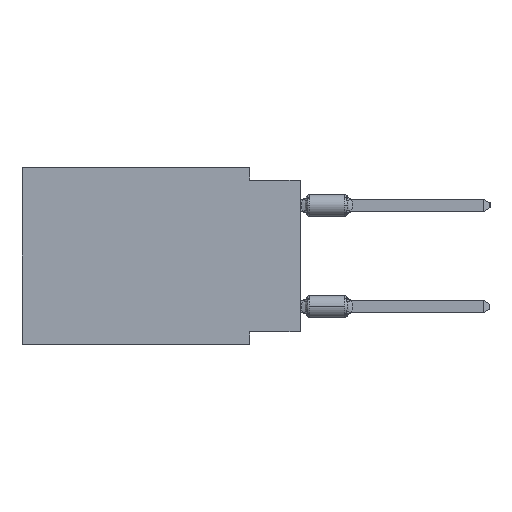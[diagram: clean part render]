
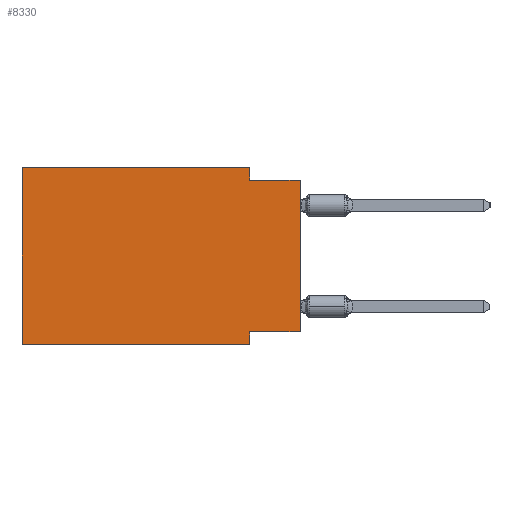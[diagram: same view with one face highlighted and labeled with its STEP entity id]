
A CAD part, left-side view. The second image highlights one B-rep face of the part: STEP entity #8330.
In plain terms, the highlighted planar face has unit normal (-1, 0, 0).
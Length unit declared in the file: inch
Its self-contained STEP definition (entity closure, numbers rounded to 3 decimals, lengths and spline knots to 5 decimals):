
#91 = LINE ( 'NONE', #12347, #8496 ) ;
#528 = VECTOR ( 'NONE', #4698, 39.37008 ) ;
#747 = ORIENTED_EDGE ( 'NONE', *, *, #12463, .F. ) ;
#889 = CARTESIAN_POINT ( 'NONE',  ( 0., 0., -0.325 ) ) ;
#1153 = VERTEX_POINT ( 'NONE', #8710 ) ;
#1393 = ORIENTED_EDGE ( 'NONE', *, *, #4732, .F. ) ;
#1495 = PLANE ( 'NONE',  #18322 ) ;
#1607 = CARTESIAN_POINT ( 'NONE',  ( 0., 0., -0.025 ) ) ;
#1635 = LINE ( 'NONE', #15175, #3743 ) ;
#1828 = CARTESIAN_POINT ( 'NONE',  ( 0., 0.1, -0.35 ) ) ;
#1936 = LINE ( 'NONE', #8005, #528 ) ;
#1984 = DIRECTION ( 'NONE',  ( 0., 0., 1. ) ) ;
#2000 = VERTEX_POINT ( 'NONE', #19093 ) ;
#2372 = CARTESIAN_POINT ( 'NONE',  ( 0., 0., -0.325 ) ) ;
#2794 = ORIENTED_EDGE ( 'NONE', *, *, #16580, .F. ) ;
#2801 = DIRECTION ( 'NONE',  ( 0., 0., -1. ) ) ;
#3112 = VERTEX_POINT ( 'NONE', #2372 ) ;
#3304 = DIRECTION ( 'NONE',  ( 0., 0., -1. ) ) ;
#3743 = VECTOR ( 'NONE', #13691, 39.37008 ) ;
#4173 = VERTEX_POINT ( 'NONE', #7600 ) ;
#4698 = DIRECTION ( 'NONE',  ( 0., 0., 1. ) ) ;
#4732 = EDGE_CURVE ( 'NONE', #1153, #16772, #4841, .T. ) ;
#4841 = LINE ( 'NONE', #10838, #7838 ) ;
#5769 = EDGE_CURVE ( 'NONE', #9960, #4173, #19409, .T. ) ;
#6175 = ORIENTED_EDGE ( 'NONE', *, *, #7003, .F. ) ;
#7003 = EDGE_CURVE ( 'NONE', #10556, #19095, #17334, .T. ) ;
#7088 = DIRECTION ( 'NONE',  ( 0., -1., 0. ) ) ;
#7468 = DIRECTION ( 'NONE',  ( 0., -1., 0. ) ) ;
#7600 = CARTESIAN_POINT ( 'NONE',  ( 0., 0.1, -0.35 ) ) ;
#7838 = VECTOR ( 'NONE', #16904, 39.37008 ) ;
#8005 = CARTESIAN_POINT ( 'NONE',  ( 0., 0., 0. ) ) ;
#8330 = ADVANCED_FACE ( 'NONE', ( #8965 ), #1495, .F. ) ;
#8496 = VECTOR ( 'NONE', #1984, 39.37008 ) ;
#8710 = CARTESIAN_POINT ( 'NONE',  ( 0., 0.55, 0. ) ) ;
#8870 = CARTESIAN_POINT ( 'NONE',  ( 0., 0.55, -0.35 ) ) ;
#8965 = FACE_OUTER_BOUND ( 'NONE', #15479, .T. ) ;
#9841 = CARTESIAN_POINT ( 'NONE',  ( 0., 0.1, -0.025 ) ) ;
#9949 = DIRECTION ( 'NONE',  ( 0., 1., 0. ) ) ;
#9960 = VERTEX_POINT ( 'NONE', #8870 ) ;
#10032 = LINE ( 'NONE', #889, #16810 ) ;
#10556 = VERTEX_POINT ( 'NONE', #9841 ) ;
#10838 = CARTESIAN_POINT ( 'NONE',  ( 0., 0.55, 0. ) ) ;
#10861 = ORIENTED_EDGE ( 'NONE', *, *, #12369, .F. ) ;
#11556 = CARTESIAN_POINT ( 'NONE',  ( 0., 0., -0.025 ) ) ;
#11732 = VECTOR ( 'NONE', #7088, 39.37008 ) ;
#11905 = ORIENTED_EDGE ( 'NONE', *, *, #18651, .T. ) ;
#12265 = ORIENTED_EDGE ( 'NONE', *, *, #5769, .T. ) ;
#12347 = CARTESIAN_POINT ( 'NONE',  ( 0., 0.55, 0. ) ) ;
#12369 = EDGE_CURVE ( 'NONE', #16772, #10556, #1635, .T. ) ;
#12463 = EDGE_CURVE ( 'NONE', #2000, #4173, #17153, .T. ) ;
#12521 = CARTESIAN_POINT ( 'NONE',  ( 0., 0.1, 0. ) ) ;
#12649 = VECTOR ( 'NONE', #3304, 39.37008 ) ;
#13460 = CARTESIAN_POINT ( 'NONE',  ( 0., 0.55, 0. ) ) ;
#13650 = CARTESIAN_POINT ( 'NONE',  ( 0., 0.55, -0.35 ) ) ;
#13691 = DIRECTION ( 'NONE',  ( 0., 0., -1. ) ) ;
#13704 = ORIENTED_EDGE ( 'NONE', *, *, #13911, .F. ) ;
#13911 = EDGE_CURVE ( 'NONE', #9960, #1153, #91, .T. ) ;
#15175 = CARTESIAN_POINT ( 'NONE',  ( 0., 0.1, 0. ) ) ;
#15479 = EDGE_LOOP ( 'NONE', ( #11905, #6175, #10861, #1393, #13704, #12265, #747, #2794 ) ) ;
#15844 = VECTOR ( 'NONE', #7468, 39.37008 ) ;
#16580 = EDGE_CURVE ( 'NONE', #3112, #2000, #10032, .T. ) ;
#16772 = VERTEX_POINT ( 'NONE', #12521 ) ;
#16810 = VECTOR ( 'NONE', #9949, 39.37008 ) ;
#16904 = DIRECTION ( 'NONE',  ( 0., -1., 0. ) ) ;
#17153 = LINE ( 'NONE', #1828, #12649 ) ;
#17334 = LINE ( 'NONE', #11556, #11732 ) ;
#18322 = AXIS2_PLACEMENT_3D ( 'NONE', #13460, #19598, #2801 ) ;
#18651 = EDGE_CURVE ( 'NONE', #3112, #19095, #1936, .T. ) ;
#19093 = CARTESIAN_POINT ( 'NONE',  ( 0., 0.1, -0.325 ) ) ;
#19095 = VERTEX_POINT ( 'NONE', #1607 ) ;
#19409 = LINE ( 'NONE', #13650, #15844 ) ;
#19598 = DIRECTION ( 'NONE',  ( 1., 0., 0. ) ) ;
